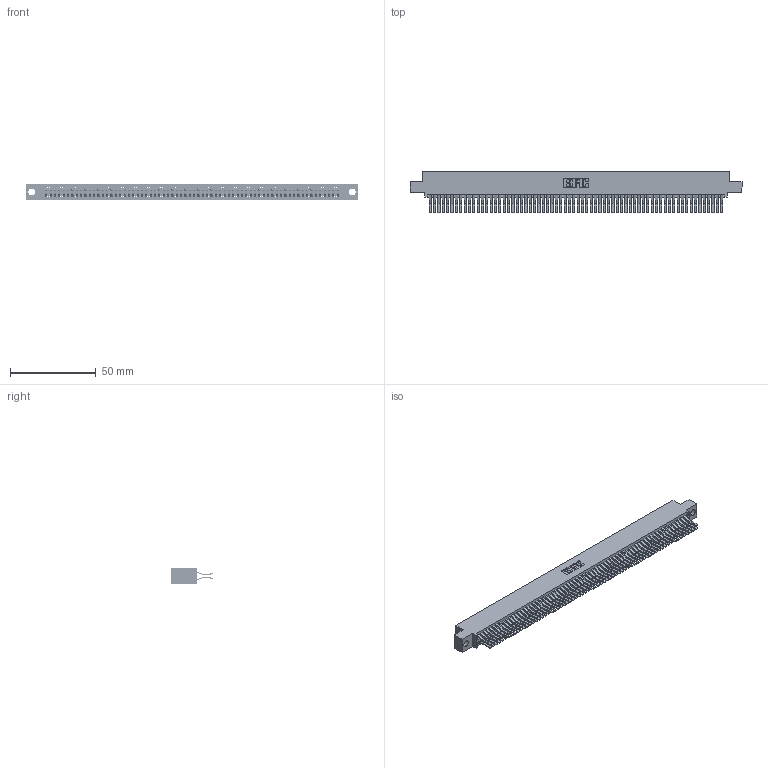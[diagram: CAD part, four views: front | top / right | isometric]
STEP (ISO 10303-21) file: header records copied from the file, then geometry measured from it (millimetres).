
FILE_DESCRIPTION (( 'STEP AP203' ), '1' );
FILE_NAME ('345-136-560-504.STEP', '2018-10-20T16:27:18', ( '' ), ( '' ), 'SwSTEP 2.0', 'SolidWorks 2016', '' );
FILE_SCHEMA (( 'CONFIG_CONTROL_DESIGN' ));
Length unit declared in the file: inch
Products named in the file (3): 345-292-001_560 Tail; 345 Part_0.110 Offset - 0.156 Dia-TH; 345-136-560-504
Assembly tree (137 placements, depth 2):
  345-136-560-504
    345 Part_0.110 Offset - 0.156 Dia-TH
    345-292-001_560 Tail  x136
Bounding box: 193.93 x 24.45 x 9.4 mm (x, y, z)
Volume: 19810 mm3; surface area: 31986.8 mm2
Topology: 137 solids, 137 shells, 7202 faces, 21433 edges, 14106 vertices
Faces by surface type: plane 4572, cylinder 2630
Entity records: 50077 total; most frequent: CARTESIAN_POINT 8372, ORIENTED_EDGE 8306, DIRECTION 7353, EDGE_CURVE 4153, LINE 3745, VECTOR 3745, VERTEX_POINT 2766, AXIS2_PLACEMENT_3D 1804
